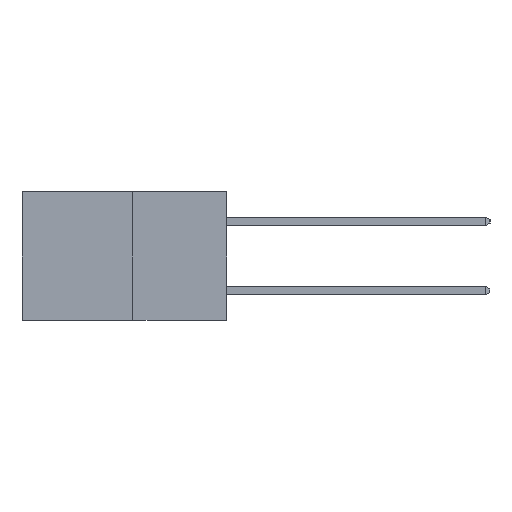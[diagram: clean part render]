
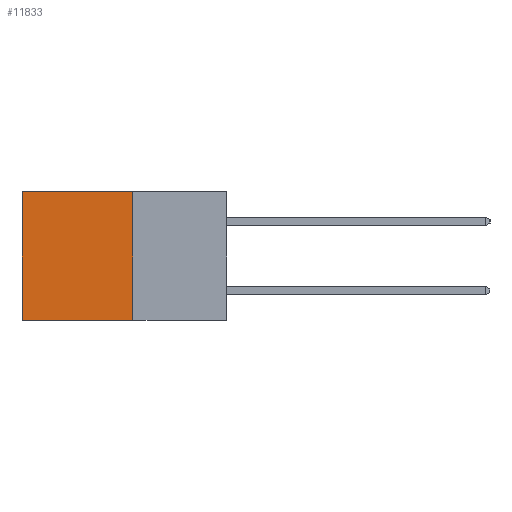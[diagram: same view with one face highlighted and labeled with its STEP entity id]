
A CAD part, left-side view. The second image highlights one B-rep face of the part: STEP entity #11833.
In plain terms, the highlighted planar face has unit normal (-1, 0, 0).
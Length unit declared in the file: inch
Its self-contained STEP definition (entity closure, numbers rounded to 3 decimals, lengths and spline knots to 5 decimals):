
#293 = VECTOR ( 'NONE', #13893, 39.37008 ) ;
#699 = CARTESIAN_POINT ( 'NONE',  ( 0.277, 0.27, -0.37 ) ) ;
#853 = CARTESIAN_POINT ( 'NONE',  ( 0.277, 0.27, -0.37 ) ) ;
#1697 = VERTEX_POINT ( 'NONE', #20375 ) ;
#2863 = VERTEX_POINT ( 'NONE', #14430 ) ;
#3369 = LINE ( 'NONE', #15019, #12758 ) ;
#3472 = ORIENTED_EDGE ( 'NONE', *, *, #11537, .F. ) ;
#3623 = DIRECTION ( 'NONE',  ( 0., 1., 0. ) ) ;
#3871 = ORIENTED_EDGE ( 'NONE', *, *, #16853, .T. ) ;
#6348 = VECTOR ( 'NONE', #17709, 39.37008 ) ;
#7213 = DIRECTION ( 'NONE',  ( 0., 0., -1. ) ) ;
#7977 = AXIS2_PLACEMENT_3D ( 'NONE', #18244, #18321, #7213 ) ;
#8870 = EDGE_LOOP ( 'NONE', ( #20274, #3472, #19501, #3871 ) ) ;
#10042 = LINE ( 'NONE', #699, #293 ) ;
#11216 = EDGE_CURVE ( 'NONE', #2863, #22205, #3369, .T. ) ;
#11421 = VECTOR ( 'NONE', #3623, 39.37008 ) ;
#11537 = EDGE_CURVE ( 'NONE', #14001, #22205, #16758, .T. ) ;
#11833 = ADVANCED_FACE ( 'NONE', ( #20195 ), #16443, .F. ) ;
#12758 = VECTOR ( 'NONE', #16869, 39.37008 ) ;
#12887 = EDGE_CURVE ( 'NONE', #1697, #14001, #10042, .T. ) ;
#13893 = DIRECTION ( 'NONE',  ( 0., 0., -1. ) ) ;
#14001 = VERTEX_POINT ( 'NONE', #20834 ) ;
#14430 = CARTESIAN_POINT ( 'NONE',  ( 0.277, 0.59, 0. ) ) ;
#14769 = CARTESIAN_POINT ( 'NONE',  ( 0.277, 0.27, 0. ) ) ;
#15019 = CARTESIAN_POINT ( 'NONE',  ( 0.277, 0.59, -0.37 ) ) ;
#15722 = LINE ( 'NONE', #14769, #11421 ) ;
#16443 = PLANE ( 'NONE',  #7977 ) ;
#16758 = LINE ( 'NONE', #853, #6348 ) ;
#16853 = EDGE_CURVE ( 'NONE', #1697, #2863, #15722, .T. ) ;
#16869 = DIRECTION ( 'NONE',  ( 0., 0., -1. ) ) ;
#17362 = CARTESIAN_POINT ( 'NONE',  ( 0.277, 0.59, -0.37 ) ) ;
#17709 = DIRECTION ( 'NONE',  ( 0., 1., 0. ) ) ;
#18244 = CARTESIAN_POINT ( 'NONE',  ( 0.277, 0.27, -0.37 ) ) ;
#18321 = DIRECTION ( 'NONE',  ( 1., 0., 0. ) ) ;
#19501 = ORIENTED_EDGE ( 'NONE', *, *, #12887, .F. ) ;
#20195 = FACE_OUTER_BOUND ( 'NONE', #8870, .T. ) ;
#20274 = ORIENTED_EDGE ( 'NONE', *, *, #11216, .T. ) ;
#20375 = CARTESIAN_POINT ( 'NONE',  ( 0.277, 0.27, 0. ) ) ;
#20834 = CARTESIAN_POINT ( 'NONE',  ( 0.277, 0.27, -0.37 ) ) ;
#22205 = VERTEX_POINT ( 'NONE', #17362 ) ;
